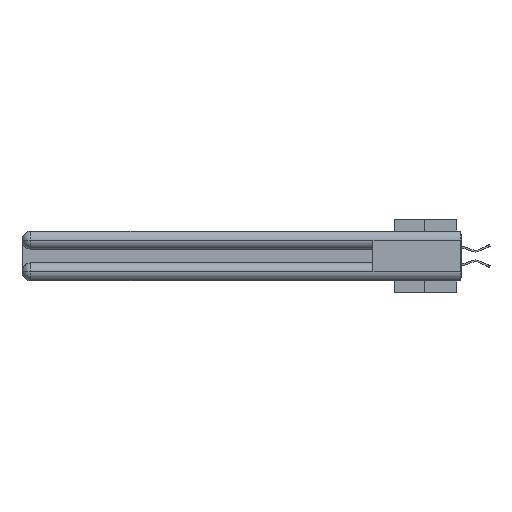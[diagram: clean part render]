
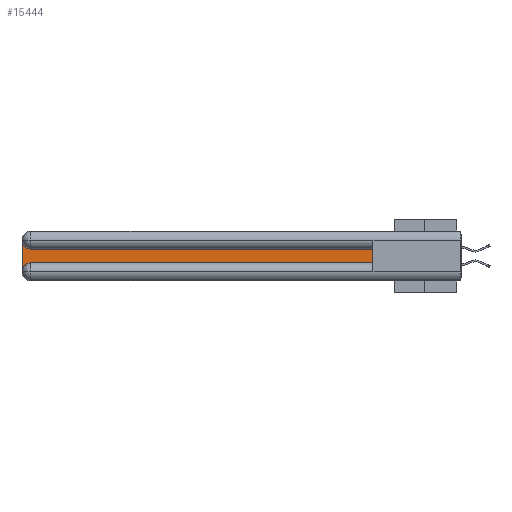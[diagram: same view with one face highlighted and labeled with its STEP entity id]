
A CAD part, left-side view. The second image highlights one B-rep face of the part: STEP entity #15444.
In plain terms, the highlighted planar face has unit normal (-1, 0, 0).
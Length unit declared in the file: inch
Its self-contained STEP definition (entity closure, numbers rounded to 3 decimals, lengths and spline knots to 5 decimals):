
#566 = ORIENTED_EDGE ( 'NONE', *, *, #20749, .T. ) ;
#1073 = ORIENTED_EDGE ( 'NONE', *, *, #4130, .T. ) ;
#1201 = CIRCLE ( 'NONE', #27734, 0.06 ) ;
#2385 = FACE_OUTER_BOUND ( 'NONE', #27329, .T. ) ;
#3731 = CARTESIAN_POINT ( 'NONE',  ( 0.075, 0.6, -0.2175 ) ) ;
#3840 = EDGE_CURVE ( 'NONE', #9188, #36307, #29018, .T. ) ;
#3871 = AXIS2_PLACEMENT_3D ( 'NONE', #16107, #4121, #7057 ) ;
#4121 = DIRECTION ( 'NONE',  ( 1., 0., 0. ) ) ;
#4130 = EDGE_CURVE ( 'NONE', #19804, #22848, #11198, .T. ) ;
#4809 = AXIS2_PLACEMENT_3D ( 'NONE', #31455, #7904, #22310 ) ;
#5060 = VECTOR ( 'NONE', #10122, 39.37008 ) ;
#5959 = EDGE_CURVE ( 'NONE', #22848, #9188, #6086, .T. ) ;
#6086 = CIRCLE ( 'NONE', #4809, 0.06 ) ;
#6551 = CARTESIAN_POINT ( 'NONE',  ( 0.075, 0.6, -0.2175 ) ) ;
#7057 = DIRECTION ( 'NONE',  ( 0., 0., -1. ) ) ;
#7904 = DIRECTION ( 'NONE',  ( 1., 0., 0. ) ) ;
#9188 = VERTEX_POINT ( 'NONE', #9443 ) ;
#9443 = CARTESIAN_POINT ( 'NONE',  ( 0.075, 2.94, -0.2175 ) ) ;
#9500 = CARTESIAN_POINT ( 'NONE',  ( 0.075, 0.6, -0.1225 ) ) ;
#10122 = DIRECTION ( 'NONE',  ( 0., 1., 0. ) ) ;
#11198 = LINE ( 'NONE', #16311, #33092 ) ;
#12039 = EDGE_CURVE ( 'NONE', #31460, #18052, #12846, .T. ) ;
#12846 = LINE ( 'NONE', #19243, #5060 ) ;
#12861 = CARTESIAN_POINT ( 'NONE',  ( 0.075, 3., -0.0625 ) ) ;
#13429 = VECTOR ( 'NONE', #21441, 39.37008 ) ;
#13556 = VECTOR ( 'NONE', #19727, 39.37008 ) ;
#15147 = DIRECTION ( 'NONE',  ( 1., 0., 0. ) ) ;
#15444 = ADVANCED_FACE ( 'NONE', ( #2385 ), #33625, .F. ) ;
#16107 = CARTESIAN_POINT ( 'NONE',  ( 0.075, 3., -0.1225 ) ) ;
#16311 = CARTESIAN_POINT ( 'NONE',  ( 0.075, 3., -0.2175 ) ) ;
#18052 = VERTEX_POINT ( 'NONE', #32959 ) ;
#19243 = CARTESIAN_POINT ( 'NONE',  ( 0.075, 0.6, -0.1225 ) ) ;
#19285 = ORIENTED_EDGE ( 'NONE', *, *, #5959, .T. ) ;
#19727 = DIRECTION ( 'NONE',  ( 0., -1., 0. ) ) ;
#19804 = VERTEX_POINT ( 'NONE', #12861 ) ;
#20749 = EDGE_CURVE ( 'NONE', #18052, #19804, #1201, .T. ) ;
#21441 = DIRECTION ( 'NONE',  ( 0., 0., 1. ) ) ;
#22310 = DIRECTION ( 'NONE',  ( 0., 0., -1. ) ) ;
#22848 = VERTEX_POINT ( 'NONE', #33421 ) ;
#27329 = EDGE_LOOP ( 'NONE', ( #28371, #566, #1073, #19285, #31904, #35142 ) ) ;
#27534 = LINE ( 'NONE', #3731, #13429 ) ;
#27734 = AXIS2_PLACEMENT_3D ( 'NONE', #32532, #15147, #35466 ) ;
#28371 = ORIENTED_EDGE ( 'NONE', *, *, #12039, .T. ) ;
#29018 = LINE ( 'NONE', #36806, #13556 ) ;
#31067 = DIRECTION ( 'NONE',  ( 0., 0., -1. ) ) ;
#31455 = CARTESIAN_POINT ( 'NONE',  ( 0.075, 2.94, -0.2775 ) ) ;
#31460 = VERTEX_POINT ( 'NONE', #9500 ) ;
#31904 = ORIENTED_EDGE ( 'NONE', *, *, #3840, .T. ) ;
#32532 = CARTESIAN_POINT ( 'NONE',  ( 0.075, 2.94, -0.0625 ) ) ;
#32959 = CARTESIAN_POINT ( 'NONE',  ( 0.075, 2.94, -0.1225 ) ) ;
#33092 = VECTOR ( 'NONE', #31067, 39.37008 ) ;
#33421 = CARTESIAN_POINT ( 'NONE',  ( 0.075, 3., -0.2775 ) ) ;
#33625 = PLANE ( 'NONE',  #3871 ) ;
#35142 = ORIENTED_EDGE ( 'NONE', *, *, #36343, .T. ) ;
#35466 = DIRECTION ( 'NONE',  ( 0., 0., -1. ) ) ;
#36307 = VERTEX_POINT ( 'NONE', #6551 ) ;
#36343 = EDGE_CURVE ( 'NONE', #36307, #31460, #27534, .T. ) ;
#36806 = CARTESIAN_POINT ( 'NONE',  ( 0.075, 0.6, -0.2175 ) ) ;
